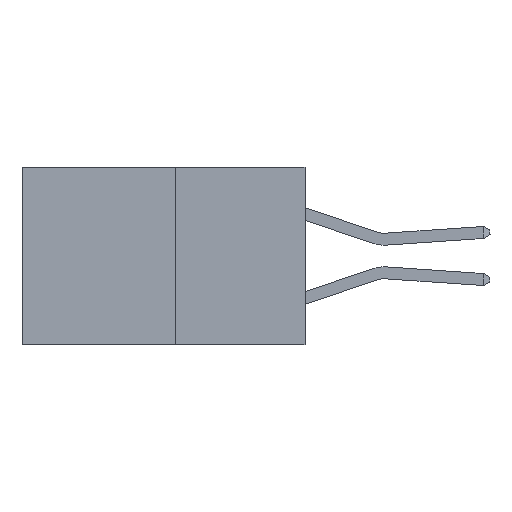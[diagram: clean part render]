
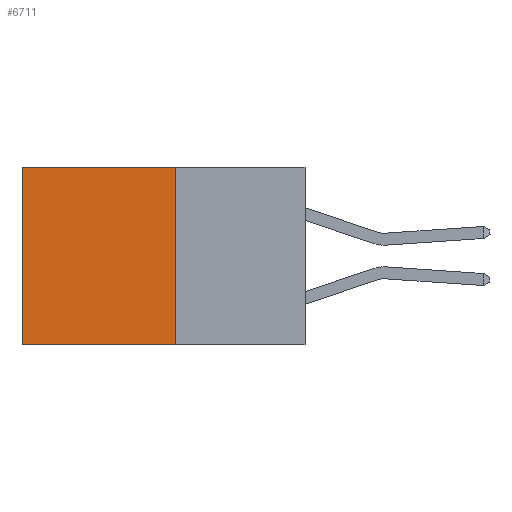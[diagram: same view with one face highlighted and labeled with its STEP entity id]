
A CAD part, left-side view. The second image highlights one B-rep face of the part: STEP entity #6711.
In plain terms, the highlighted planar face has unit normal (-1, 0, 0).
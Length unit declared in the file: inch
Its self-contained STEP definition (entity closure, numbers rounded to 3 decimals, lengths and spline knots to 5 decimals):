
#8 = CARTESIAN_POINT ( 'NONE',  ( 0.277, 0.59, -0.37 ) ) ;
#172 = VECTOR ( 'NONE', #8724, 39.37008 ) ;
#1327 = VECTOR ( 'NONE', #9321, 39.37008 ) ;
#1579 = CARTESIAN_POINT ( 'NONE',  ( 0.277, 0.27, -0.37 ) ) ;
#1905 = PLANE ( 'NONE',  #15584 ) ;
#2646 = CARTESIAN_POINT ( 'NONE',  ( 0.277, 0.59, -0.37 ) ) ;
#2864 = EDGE_CURVE ( 'NONE', #16853, #8463, #5086, .T. ) ;
#3291 = DIRECTION ( 'NONE',  ( 0., 0., -1. ) ) ;
#4761 = LINE ( 'NONE', #2646, #11730 ) ;
#5086 = LINE ( 'NONE', #13302, #1327 ) ;
#5651 = CARTESIAN_POINT ( 'NONE',  ( 0.277, 0.59, 0. ) ) ;
#5799 = CARTESIAN_POINT ( 'NONE',  ( 0.277, 0.27, 0. ) ) ;
#6380 = LINE ( 'NONE', #1579, #12901 ) ;
#6691 = FACE_OUTER_BOUND ( 'NONE', #15303, .T. ) ;
#6711 = ADVANCED_FACE ( 'NONE', ( #6691 ), #1905, .F. ) ;
#7145 = VERTEX_POINT ( 'NONE', #16834 ) ;
#7830 = ORIENTED_EDGE ( 'NONE', *, *, #8486, .F. ) ;
#8463 = VERTEX_POINT ( 'NONE', #8 ) ;
#8486 = EDGE_CURVE ( 'NONE', #7145, #16853, #6380, .T. ) ;
#8724 = DIRECTION ( 'NONE',  ( 0., 1., 0. ) ) ;
#9282 = EDGE_CURVE ( 'NONE', #7145, #16980, #11373, .T. ) ;
#9321 = DIRECTION ( 'NONE',  ( 0., 1., 0. ) ) ;
#9524 = CARTESIAN_POINT ( 'NONE',  ( 0.277, 0.27, -0.37 ) ) ;
#9969 = DIRECTION ( 'NONE',  ( 0., 0., -1. ) ) ;
#11076 = EDGE_CURVE ( 'NONE', #16980, #8463, #4761, .T. ) ;
#11373 = LINE ( 'NONE', #5799, #172 ) ;
#11699 = DIRECTION ( 'NONE',  ( 1., 0., 0. ) ) ;
#11730 = VECTOR ( 'NONE', #15177, 39.37008 ) ;
#12901 = VECTOR ( 'NONE', #9969, 39.37008 ) ;
#13291 = ORIENTED_EDGE ( 'NONE', *, *, #2864, .F. ) ;
#13302 = CARTESIAN_POINT ( 'NONE',  ( 0.277, 0.27, -0.37 ) ) ;
#15177 = DIRECTION ( 'NONE',  ( 0., 0., -1. ) ) ;
#15239 = ORIENTED_EDGE ( 'NONE', *, *, #11076, .T. ) ;
#15303 = EDGE_LOOP ( 'NONE', ( #15239, #13291, #7830, #17546 ) ) ;
#15584 = AXIS2_PLACEMENT_3D ( 'NONE', #17079, #11699, #3291 ) ;
#16834 = CARTESIAN_POINT ( 'NONE',  ( 0.277, 0.27, 0. ) ) ;
#16853 = VERTEX_POINT ( 'NONE', #9524 ) ;
#16980 = VERTEX_POINT ( 'NONE', #5651 ) ;
#17079 = CARTESIAN_POINT ( 'NONE',  ( 0.277, 0.27, -0.37 ) ) ;
#17546 = ORIENTED_EDGE ( 'NONE', *, *, #9282, .T. ) ;
